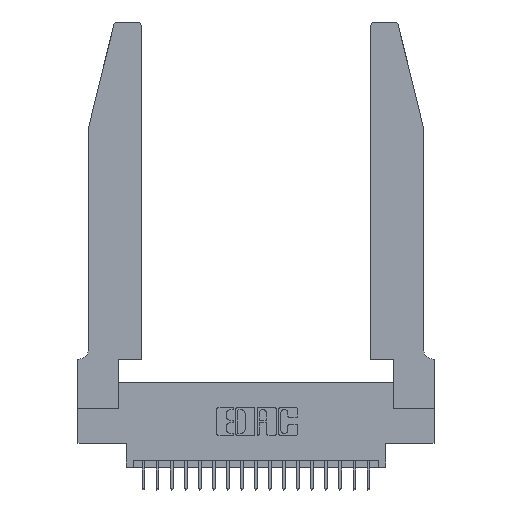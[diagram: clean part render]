
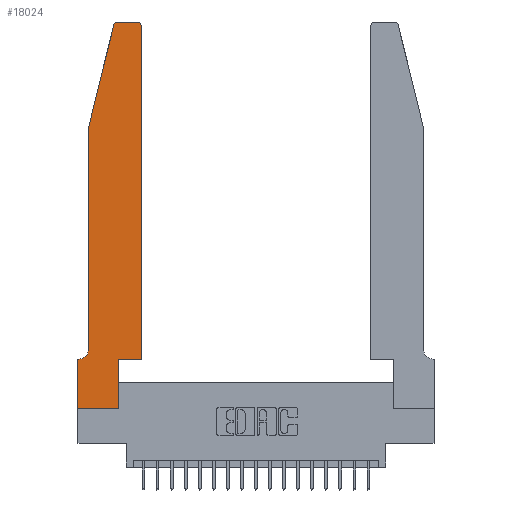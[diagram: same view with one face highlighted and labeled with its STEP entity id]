
A CAD part, top view. The second image highlights one B-rep face of the part: STEP entity #18024.
In plain terms, the highlighted planar face has unit normal (0, 0, 1).
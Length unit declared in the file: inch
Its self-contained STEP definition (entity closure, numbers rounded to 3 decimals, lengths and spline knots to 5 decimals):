
#303 = VECTOR ( 'NONE', #9431, 39.37008 ) ;
#467 = CARTESIAN_POINT ( 'NONE',  ( 0.0755, 2., 0.37 ) ) ;
#479 = VECTOR ( 'NONE', #11458, 39.37008 ) ;
#935 = VECTOR ( 'NONE', #11767, 39.37008 ) ;
#1010 = ORIENTED_EDGE ( 'NONE', *, *, #16600, .T. ) ;
#1172 = AXIS2_PLACEMENT_3D ( 'NONE', #1912, #11899, #5108 ) ;
#1208 = AXIS2_PLACEMENT_3D ( 'NONE', #17130, #15429, #5241 ) ;
#1330 = EDGE_CURVE ( 'NONE', #7184, #4315, #21686, .T. ) ;
#1340 = LINE ( 'NONE', #12054, #8899 ) ;
#1437 = CARTESIAN_POINT ( 'NONE',  ( 0.284, 2.75, 0.37 ) ) ;
#1516 = EDGE_CURVE ( 'NONE', #17592, #15388, #3640, .T. ) ;
#1535 = LINE ( 'NONE', #7859, #479 ) ;
#1912 = CARTESIAN_POINT ( 'NONE',  ( 0.0055, 0.42, 0.37 ) ) ;
#2142 = DIRECTION ( 'NONE',  ( 0., -1., 0. ) ) ;
#2649 = ORIENTED_EDGE ( 'NONE', *, *, #16573, .T. ) ;
#2841 = CARTESIAN_POINT ( 'NONE',  ( 0.4205, 2.75, 0.37 ) ) ;
#3253 = EDGE_CURVE ( 'NONE', #4315, #7327, #14308, .T. ) ;
#3589 = DIRECTION ( 'NONE',  ( 0., 0., 1. ) ) ;
#3640 = LINE ( 'NONE', #20435, #19894 ) ;
#3750 = EDGE_LOOP ( 'NONE', ( #2649, #1010, #17695, #9146, #17026, #18379, #13563, #21411, #20026, #11779, #9124, #9917 ) ) ;
#4093 = CARTESIAN_POINT ( 'NONE',  ( 0., 0., 0.37 ) ) ;
#4226 = EDGE_CURVE ( 'NONE', #10896, #17269, #1340, .T. ) ;
#4315 = VERTEX_POINT ( 'NONE', #7852 ) ;
#4357 = CARTESIAN_POINT ( 'NONE',  ( 0.0055, 0.35, 0.37 ) ) ;
#4765 = EDGE_CURVE ( 'NONE', #7327, #17592, #7068, .T. ) ;
#5108 = DIRECTION ( 'NONE',  ( -1., 0., 0. ) ) ;
#5241 = DIRECTION ( 'NONE',  ( 1., 0., 0. ) ) ;
#5253 = CARTESIAN_POINT ( 'NONE',  ( 0.284, 2.72, 0.37 ) ) ;
#5315 = EDGE_CURVE ( 'NONE', #17336, #10896, #1535, .T. ) ;
#5344 = CARTESIAN_POINT ( 'NONE',  ( 0.4505, 2.72, 0.37 ) ) ;
#6611 = DIRECTION ( 'NONE',  ( 1., 0., 0. ) ) ;
#6739 = EDGE_CURVE ( 'NONE', #9992, #13620, #19376, .T. ) ;
#6930 = CARTESIAN_POINT ( 'NONE',  ( 0.4505, 0.35, 0.37 ) ) ;
#7068 = CIRCLE ( 'NONE', #1172, 0.07 ) ;
#7090 = VECTOR ( 'NONE', #6611, 39.37008 ) ;
#7184 = VERTEX_POINT ( 'NONE', #20585 ) ;
#7327 = VERTEX_POINT ( 'NONE', #19365 ) ;
#7852 = CARTESIAN_POINT ( 'NONE',  ( 0.0755, 2., 0.37 ) ) ;
#7859 = CARTESIAN_POINT ( 'NONE',  ( 0., 0., 0.37 ) ) ;
#8192 = VECTOR ( 'NONE', #15143, 39.37008 ) ;
#8704 = CIRCLE ( 'NONE', #8993, 0.03 ) ;
#8757 = CARTESIAN_POINT ( 'NONE',  ( 0., 0.35, 0.37 ) ) ;
#8899 = VECTOR ( 'NONE', #17282, 39.37008 ) ;
#8993 = AXIS2_PLACEMENT_3D ( 'NONE', #5253, #3589, #13769 ) ;
#9124 = ORIENTED_EDGE ( 'NONE', *, *, #12163, .T. ) ;
#9146 = ORIENTED_EDGE ( 'NONE', *, *, #3253, .T. ) ;
#9431 = DIRECTION ( 'NONE',  ( 0., 1., 0. ) ) ;
#9462 = DIRECTION ( 'NONE',  ( -1., 0., 0. ) ) ;
#9917 = ORIENTED_EDGE ( 'NONE', *, *, #6739, .T. ) ;
#9966 = LINE ( 'NONE', #10776, #303 ) ;
#9992 = VERTEX_POINT ( 'NONE', #5344 ) ;
#10294 = FACE_OUTER_BOUND ( 'NONE', #3750, .T. ) ;
#10617 = VECTOR ( 'NONE', #2142, 39.37008 ) ;
#10669 = VERTEX_POINT ( 'NONE', #6930 ) ;
#10776 = CARTESIAN_POINT ( 'NONE',  ( 0.4505, 0.35, 0.37 ) ) ;
#10896 = VERTEX_POINT ( 'NONE', #19108 ) ;
#11411 = CARTESIAN_POINT ( 'NONE',  ( 0.4505, 0.35, 0.37 ) ) ;
#11458 = DIRECTION ( 'NONE',  ( 1., 0., 0. ) ) ;
#11767 = DIRECTION ( 'NONE',  ( -1., 0., 0. ) ) ;
#11779 = ORIENTED_EDGE ( 'NONE', *, *, #12615, .T. ) ;
#11888 = CARTESIAN_POINT ( 'NONE',  ( 0., 0.35, 0.37 ) ) ;
#11899 = DIRECTION ( 'NONE',  ( 0., 0., -1. ) ) ;
#12054 = CARTESIAN_POINT ( 'NONE',  ( 0.2865, 0.35, 0.37 ) ) ;
#12163 = EDGE_CURVE ( 'NONE', #10669, #9992, #9966, .T. ) ;
#12179 = LINE ( 'NONE', #20217, #935 ) ;
#12615 = EDGE_CURVE ( 'NONE', #17269, #10669, #18662, .T. ) ;
#12709 = LINE ( 'NONE', #15449, #8192 ) ;
#12852 = AXIS2_PLACEMENT_3D ( 'NONE', #8757, #18709, #17321 ) ;
#13563 = ORIENTED_EDGE ( 'NONE', *, *, #16568, .T. ) ;
#13620 = VERTEX_POINT ( 'NONE', #2841 ) ;
#13769 = DIRECTION ( 'NONE',  ( 1., 0., 0. ) ) ;
#14308 = LINE ( 'NONE', #17094, #10617 ) ;
#15143 = DIRECTION ( 'NONE',  ( 0., -1., 0. ) ) ;
#15388 = VERTEX_POINT ( 'NONE', #11888 ) ;
#15429 = DIRECTION ( 'NONE',  ( 0., 0., 1. ) ) ;
#15449 = CARTESIAN_POINT ( 'NONE',  ( 0., 0., 0.37 ) ) ;
#16568 = EDGE_CURVE ( 'NONE', #15388, #17336, #12709, .T. ) ;
#16573 = EDGE_CURVE ( 'NONE', #13620, #20633, #12179, .T. ) ;
#16600 = EDGE_CURVE ( 'NONE', #20633, #7184, #8704, .T. ) ;
#16970 = CARTESIAN_POINT ( 'NONE',  ( 0.2865, 0.35, 0.37 ) ) ;
#17026 = ORIENTED_EDGE ( 'NONE', *, *, #4765, .T. ) ;
#17094 = CARTESIAN_POINT ( 'NONE',  ( 0.0755, 2., 0.37 ) ) ;
#17130 = CARTESIAN_POINT ( 'NONE',  ( 0.4205, 2.72, 0.37 ) ) ;
#17166 = PLANE ( 'NONE',  #12852 ) ;
#17269 = VERTEX_POINT ( 'NONE', #16970 ) ;
#17282 = DIRECTION ( 'NONE',  ( 0., 1., 0. ) ) ;
#17321 = DIRECTION ( 'NONE',  ( 1., 0., 0. ) ) ;
#17336 = VERTEX_POINT ( 'NONE', #4093 ) ;
#17548 = VECTOR ( 'NONE', #20550, 39.37008 ) ;
#17592 = VERTEX_POINT ( 'NONE', #4357 ) ;
#17695 = ORIENTED_EDGE ( 'NONE', *, *, #1330, .T. ) ;
#18024 = ADVANCED_FACE ( 'NONE', ( #10294 ), #17166, .T. ) ;
#18379 = ORIENTED_EDGE ( 'NONE', *, *, #1516, .T. ) ;
#18662 = LINE ( 'NONE', #11411, #7090 ) ;
#18709 = DIRECTION ( 'NONE',  ( 0., 0., 1. ) ) ;
#19108 = CARTESIAN_POINT ( 'NONE',  ( 0.2865, 0., 0.37 ) ) ;
#19365 = CARTESIAN_POINT ( 'NONE',  ( 0.0755, 0.42, 0.37 ) ) ;
#19376 = CIRCLE ( 'NONE', #1208, 0.03 ) ;
#19894 = VECTOR ( 'NONE', #9462, 39.37008 ) ;
#20026 = ORIENTED_EDGE ( 'NONE', *, *, #4226, .T. ) ;
#20217 = CARTESIAN_POINT ( 'NONE',  ( 0.2605, 2.75, 0.37 ) ) ;
#20435 = CARTESIAN_POINT ( 'NONE',  ( 0.0755, 0.35, 0.37 ) ) ;
#20550 = DIRECTION ( 'NONE',  ( -0.239, -0.971, 0. ) ) ;
#20585 = CARTESIAN_POINT ( 'NONE',  ( 0.25487, 2.72718, 0.37 ) ) ;
#20633 = VERTEX_POINT ( 'NONE', #1437 ) ;
#21411 = ORIENTED_EDGE ( 'NONE', *, *, #5315, .T. ) ;
#21686 = LINE ( 'NONE', #467, #17548 ) ;
